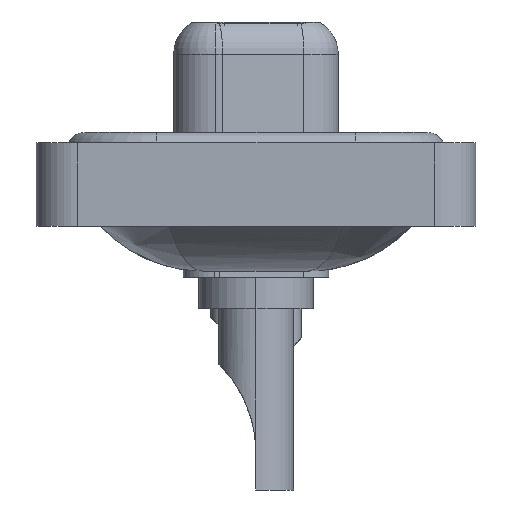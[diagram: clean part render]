
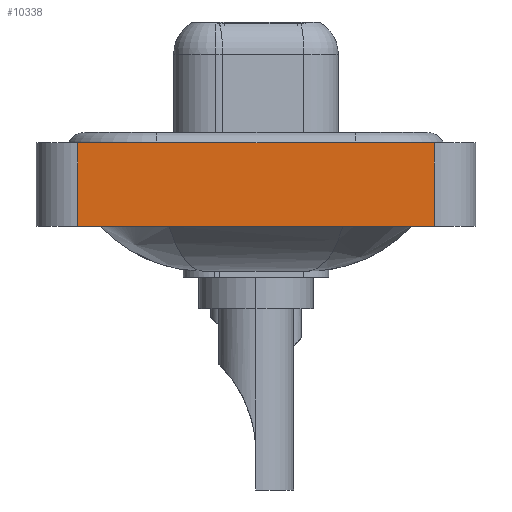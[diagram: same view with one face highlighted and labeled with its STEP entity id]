
A CAD part, left-side view. The second image highlights one B-rep face of the part: STEP entity #10338.
In plain terms, the highlighted planar face has unit normal (-1, 0, 0).
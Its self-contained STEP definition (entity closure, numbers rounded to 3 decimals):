
#383 = DIRECTION ( 'NONE',  ( 0., 0., 1. ) ) ;
#645 = CARTESIAN_POINT ( 'NONE',  ( -7.3, 8.55, -3.6 ) ) ;
#768 = AXIS2_PLACEMENT_3D ( 'NONE', #13039, #11475, #383 ) ;
#856 = ORIENTED_EDGE ( 'NONE', *, *, #18905, .F. ) ;
#978 = CARTESIAN_POINT ( 'NONE',  ( -7.3, 8.55, -3.6 ) ) ;
#1073 = ORIENTED_EDGE ( 'NONE', *, *, #15065, .T. ) ;
#1779 = VECTOR ( 'NONE', #17725, 1000. ) ;
#3347 = CARTESIAN_POINT ( 'NONE',  ( -7.3, -8.55, -3.6 ) ) ;
#3439 = LINE ( 'NONE', #3347, #1779 ) ;
#3516 = ORIENTED_EDGE ( 'NONE', *, *, #19279, .T. ) ;
#5060 = CARTESIAN_POINT ( 'NONE',  ( -7.3, -8.55, -3.6 ) ) ;
#5267 = DIRECTION ( 'NONE',  ( 0., 0., 1. ) ) ;
#5807 = DIRECTION ( 'NONE',  ( 0., 0., 1. ) ) ;
#6245 = DIRECTION ( 'NONE',  ( 0., -1., 0. ) ) ;
#7795 = LINE ( 'NONE', #20482, #8014 ) ;
#8014 = VECTOR ( 'NONE', #6245, 1000. ) ;
#9775 = VERTEX_POINT ( 'NONE', #14713 ) ;
#10010 = FACE_OUTER_BOUND ( 'NONE', #20315, .T. ) ;
#10338 = ADVANCED_FACE ( 'NONE', ( #10010 ), #18015, .T. ) ;
#10397 = LINE ( 'NONE', #978, #19958 ) ;
#10530 = VERTEX_POINT ( 'NONE', #18422 ) ;
#11475 = DIRECTION ( 'NONE',  ( -1., 0., 0. ) ) ;
#13039 = CARTESIAN_POINT ( 'NONE',  ( -7.3, -8.55, -3.6 ) ) ;
#14016 = VECTOR ( 'NONE', #5267, 1000. ) ;
#14713 = CARTESIAN_POINT ( 'NONE',  ( -7.3, -8.55, 0.4 ) ) ;
#15065 = EDGE_CURVE ( 'NONE', #19424, #10530, #3439, .T. ) ;
#16345 = CARTESIAN_POINT ( 'NONE',  ( -7.3, 8.55, 0.4 ) ) ;
#17112 = ORIENTED_EDGE ( 'NONE', *, *, #19170, .F. ) ;
#17725 = DIRECTION ( 'NONE',  ( 0., -1., 0. ) ) ;
#18015 = PLANE ( 'NONE',  #768 ) ;
#18126 = VERTEX_POINT ( 'NONE', #16345 ) ;
#18422 = CARTESIAN_POINT ( 'NONE',  ( -7.3, -8.55, -3.6 ) ) ;
#18905 = EDGE_CURVE ( 'NONE', #19424, #18126, #10397, .T. ) ;
#19170 = EDGE_CURVE ( 'NONE', #18126, #9775, #7795, .T. ) ;
#19226 = LINE ( 'NONE', #5060, #14016 ) ;
#19279 = EDGE_CURVE ( 'NONE', #10530, #9775, #19226, .T. ) ;
#19424 = VERTEX_POINT ( 'NONE', #645 ) ;
#19958 = VECTOR ( 'NONE', #5807, 1000. ) ;
#20315 = EDGE_LOOP ( 'NONE', ( #3516, #17112, #856, #1073 ) ) ;
#20482 = CARTESIAN_POINT ( 'NONE',  ( -7.3, -8.55, 0.4 ) ) ;
